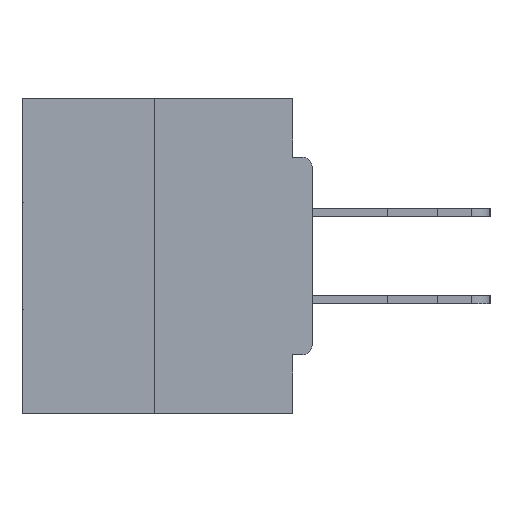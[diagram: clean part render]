
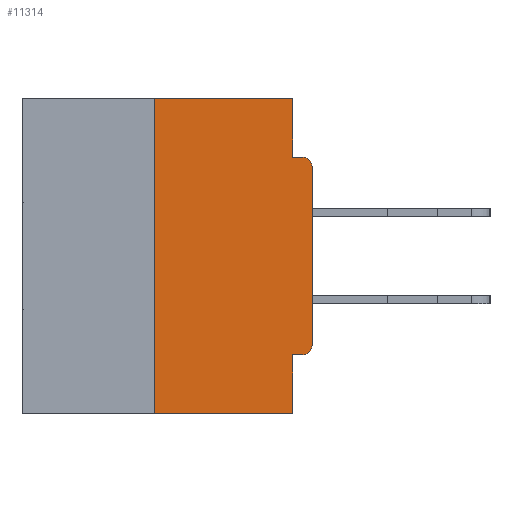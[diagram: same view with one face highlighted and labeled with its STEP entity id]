
A CAD part, left-side view. The second image highlights one B-rep face of the part: STEP entity #11314.
In plain terms, the highlighted planar face has unit normal (-1, 0, 0).
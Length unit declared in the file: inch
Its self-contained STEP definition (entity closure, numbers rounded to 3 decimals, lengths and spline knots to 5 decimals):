
#93 = EDGE_CURVE ( 'NONE', #13658, #2284, #32933, .T. ) ;
#106 = CARTESIAN_POINT ( 'NONE',  ( 0., 0.015, -0.4065 ) ) ;
#446 = ORIENTED_EDGE ( 'NONE', *, *, #93, .F. ) ;
#467 = DIRECTION ( 'NONE',  ( 0., 1., 0. ) ) ;
#615 = CARTESIAN_POINT ( 'NONE',  ( 0., 0.031, -0.5 ) ) ;
#700 = EDGE_CURVE ( 'NONE', #2284, #31451, #18914, .T. ) ;
#1236 = ORIENTED_EDGE ( 'NONE', *, *, #15437, .F. ) ;
#1323 = CARTESIAN_POINT ( 'NONE',  ( 0., 0.46, 0. ) ) ;
#1726 = ORIENTED_EDGE ( 'NONE', *, *, #8092, .T. ) ;
#2284 = VERTEX_POINT ( 'NONE', #19759 ) ;
#2584 = DIRECTION ( 'NONE',  ( 0., 0., 1. ) ) ;
#2745 = DIRECTION ( 'NONE',  ( -1., 0., 0. ) ) ;
#2812 = AXIS2_PLACEMENT_3D ( 'NONE', #17841, #2745, #24283 ) ;
#3828 = LINE ( 'NONE', #37505, #31823 ) ;
#4403 = DIRECTION ( 'NONE',  ( 0., 0., -1. ) ) ;
#4435 = VERTEX_POINT ( 'NONE', #35798 ) ;
#4643 = EDGE_CURVE ( 'NONE', #33925, #12430, #8252, .T. ) ;
#4882 = DIRECTION ( 'NONE',  ( 0., 0., -1. ) ) ;
#5113 = EDGE_CURVE ( 'NONE', #4435, #22341, #34316, .T. ) ;
#5140 = VECTOR ( 'NONE', #7105, 39.37008 ) ;
#5229 = CARTESIAN_POINT ( 'NONE',  ( 0., 0.46, 0. ) ) ;
#5891 = VECTOR ( 'NONE', #17510, 39.37008 ) ;
#6104 = AXIS2_PLACEMENT_3D ( 'NONE', #38576, #32799, #4882 ) ;
#6723 = CARTESIAN_POINT ( 'NONE',  ( 0., 0., -0.3915 ) ) ;
#7105 = DIRECTION ( 'NONE',  ( 0., -1., 0. ) ) ;
#7484 = CARTESIAN_POINT ( 'NONE',  ( 0., 0.031, -0.0935 ) ) ;
#8092 = EDGE_CURVE ( 'NONE', #13658, #37525, #38417, .T. ) ;
#8179 = VECTOR ( 'NONE', #10140, 39.37008 ) ;
#8252 = LINE ( 'NONE', #25007, #14063 ) ;
#8393 = CARTESIAN_POINT ( 'NONE',  ( 0., 0.031, 0. ) ) ;
#9113 = CARTESIAN_POINT ( 'NONE',  ( 0., 0.25, -0.5 ) ) ;
#9766 = DIRECTION ( 'NONE',  ( 0., 0., -1. ) ) ;
#9967 = VERTEX_POINT ( 'NONE', #6723 ) ;
#10140 = DIRECTION ( 'NONE',  ( 0., -1., 0. ) ) ;
#10962 = AXIS2_PLACEMENT_3D ( 'NONE', #1323, #20039, #4403 ) ;
#11099 = LINE ( 'NONE', #28600, #8179 ) ;
#11314 = ADVANCED_FACE ( 'NONE', ( #22709 ), #35386, .F. ) ;
#12151 = EDGE_LOOP ( 'NONE', ( #13187, #446, #1726, #1236, #25235, #16934, #34672, #17464, #16385, #20777 ) ) ;
#12304 = EDGE_CURVE ( 'NONE', #31451, #23505, #3828, .T. ) ;
#12430 = VERTEX_POINT ( 'NONE', #29009 ) ;
#12447 = CIRCLE ( 'NONE', #6104, 0.015 ) ;
#13187 = ORIENTED_EDGE ( 'NONE', *, *, #700, .F. ) ;
#13658 = VERTEX_POINT ( 'NONE', #9113 ) ;
#14048 = CARTESIAN_POINT ( 'NONE',  ( 0., 0.25, 0. ) ) ;
#14054 = EDGE_CURVE ( 'NONE', #33925, #9967, #12447, .T. ) ;
#14063 = VECTOR ( 'NONE', #467, 39.37008 ) ;
#14810 = VECTOR ( 'NONE', #25670, 39.37008 ) ;
#15136 = EDGE_CURVE ( 'NONE', #23505, #22341, #11099, .T. ) ;
#15437 = EDGE_CURVE ( 'NONE', #12430, #37525, #31294, .T. ) ;
#16385 = ORIENTED_EDGE ( 'NONE', *, *, #15136, .F. ) ;
#16934 = ORIENTED_EDGE ( 'NONE', *, *, #14054, .T. ) ;
#17403 = EDGE_CURVE ( 'NONE', #9967, #4435, #37446, .T. ) ;
#17464 = ORIENTED_EDGE ( 'NONE', *, *, #5113, .T. ) ;
#17510 = DIRECTION ( 'NONE',  ( 0., -1., 0. ) ) ;
#17841 = CARTESIAN_POINT ( 'NONE',  ( 0., 0.015, -0.1085 ) ) ;
#18914 = LINE ( 'NONE', #5229, #5891 ) ;
#19759 = CARTESIAN_POINT ( 'NONE',  ( 0., 0.25, 0. ) ) ;
#20039 = DIRECTION ( 'NONE',  ( 1., 0., 0. ) ) ;
#20777 = ORIENTED_EDGE ( 'NONE', *, *, #12304, .F. ) ;
#22323 = VECTOR ( 'NONE', #2584, 39.37008 ) ;
#22341 = VERTEX_POINT ( 'NONE', #24765 ) ;
#22709 = FACE_OUTER_BOUND ( 'NONE', #12151, .T. ) ;
#23100 = VECTOR ( 'NONE', #35986, 39.37008 ) ;
#23505 = VERTEX_POINT ( 'NONE', #7484 ) ;
#24283 = DIRECTION ( 'NONE',  ( 0., 0., -1. ) ) ;
#24765 = CARTESIAN_POINT ( 'NONE',  ( 0., 0.015, -0.0935 ) ) ;
#25007 = CARTESIAN_POINT ( 'NONE',  ( 0., 0., -0.4065 ) ) ;
#25235 = ORIENTED_EDGE ( 'NONE', *, *, #4643, .F. ) ;
#25670 = DIRECTION ( 'NONE',  ( 0., 0., 1. ) ) ;
#28600 = CARTESIAN_POINT ( 'NONE',  ( 0., 0., -0.0935 ) ) ;
#29009 = CARTESIAN_POINT ( 'NONE',  ( 0., 0.031, -0.4065 ) ) ;
#29798 = CARTESIAN_POINT ( 'NONE',  ( 0., 0.031, -0.5 ) ) ;
#31294 = LINE ( 'NONE', #29798, #23100 ) ;
#31451 = VERTEX_POINT ( 'NONE', #8393 ) ;
#31823 = VECTOR ( 'NONE', #9766, 39.37008 ) ;
#32042 = CARTESIAN_POINT ( 'NONE',  ( 0., 0.46, -0.5 ) ) ;
#32147 = CARTESIAN_POINT ( 'NONE',  ( 0., 0., 0. ) ) ;
#32799 = DIRECTION ( 'NONE',  ( -1., 0., 0. ) ) ;
#32933 = LINE ( 'NONE', #14048, #22323 ) ;
#33925 = VERTEX_POINT ( 'NONE', #106 ) ;
#34316 = CIRCLE ( 'NONE', #2812, 0.015 ) ;
#34672 = ORIENTED_EDGE ( 'NONE', *, *, #17403, .T. ) ;
#35386 = PLANE ( 'NONE',  #10962 ) ;
#35798 = CARTESIAN_POINT ( 'NONE',  ( 0., 0., -0.1085 ) ) ;
#35986 = DIRECTION ( 'NONE',  ( 0., 0., -1. ) ) ;
#37446 = LINE ( 'NONE', #32147, #14810 ) ;
#37505 = CARTESIAN_POINT ( 'NONE',  ( 0., 0.031, 0. ) ) ;
#37525 = VERTEX_POINT ( 'NONE', #615 ) ;
#38417 = LINE ( 'NONE', #32042, #5140 ) ;
#38576 = CARTESIAN_POINT ( 'NONE',  ( 0., 0.015, -0.3915 ) ) ;
